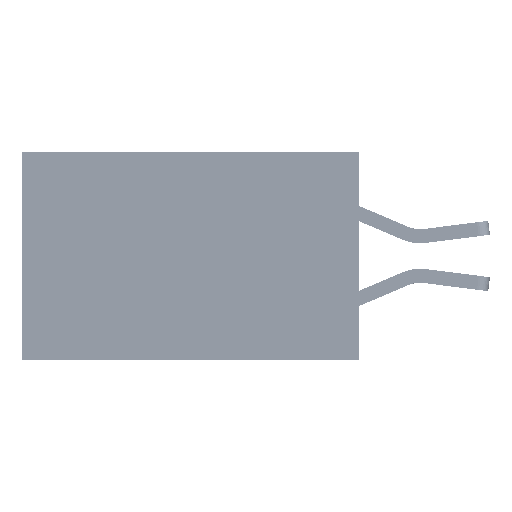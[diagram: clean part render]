
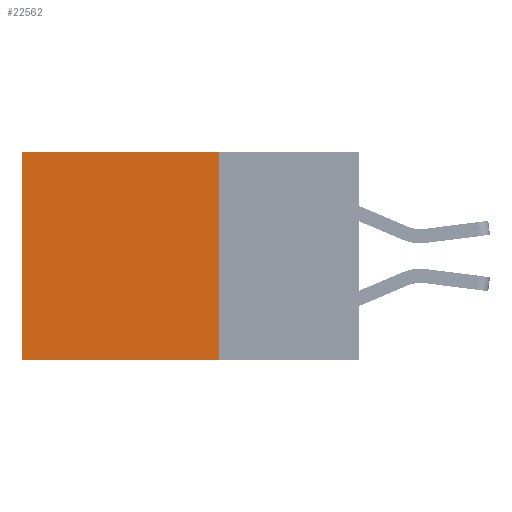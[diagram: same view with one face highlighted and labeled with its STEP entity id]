
A CAD part, left-side view. The second image highlights one B-rep face of the part: STEP entity #22562.
In plain terms, the highlighted planar face has unit normal (-1, 0, 0).
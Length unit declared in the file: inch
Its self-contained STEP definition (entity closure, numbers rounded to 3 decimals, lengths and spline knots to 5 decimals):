
#1526 = AXIS2_PLACEMENT_3D ( 'NONE', #34765, #31621, #42800 ) ;
#2693 = CARTESIAN_POINT ( 'NONE',  ( 0.2875, 0.6, -0.37 ) ) ;
#3317 = LINE ( 'NONE', #44154, #21905 ) ;
#4428 = LINE ( 'NONE', #11513, #46806 ) ;
#4914 = DIRECTION ( 'NONE',  ( 0., 1., 0. ) ) ;
#7636 = VERTEX_POINT ( 'NONE', #46357 ) ;
#10090 = ORIENTED_EDGE ( 'NONE', *, *, #46608, .F. ) ;
#11513 = CARTESIAN_POINT ( 'NONE',  ( 0.2875, 0.25, 0. ) ) ;
#11705 = EDGE_CURVE ( 'NONE', #7636, #19095, #32426, .T. ) ;
#14735 = LINE ( 'NONE', #37545, #40987 ) ;
#15252 = CARTESIAN_POINT ( 'NONE',  ( 0.2875, 0.25, -0.37 ) ) ;
#18324 = ORIENTED_EDGE ( 'NONE', *, *, #11705, .T. ) ;
#18433 = VERTEX_POINT ( 'NONE', #15252 ) ;
#19095 = VERTEX_POINT ( 'NONE', #2693 ) ;
#21905 = VECTOR ( 'NONE', #32981, 39.37008 ) ;
#22562 = ADVANCED_FACE ( 'NONE', ( #23873 ), #35494, .F. ) ;
#23577 = VECTOR ( 'NONE', #43610, 39.37008 ) ;
#23873 = FACE_OUTER_BOUND ( 'NONE', #39299, .T. ) ;
#30512 = DIRECTION ( 'NONE',  ( 0., 0., -1. ) ) ;
#31621 = DIRECTION ( 'NONE',  ( 1., 0., 0. ) ) ;
#32426 = LINE ( 'NONE', #47959, #23577 ) ;
#32981 = DIRECTION ( 'NONE',  ( 0., 1., 0. ) ) ;
#34765 = CARTESIAN_POINT ( 'NONE',  ( 0.2875, 0.25, 0. ) ) ;
#35494 = PLANE ( 'NONE',  #1526 ) ;
#35618 = EDGE_CURVE ( 'NONE', #18433, #19095, #3317, .T. ) ;
#37545 = CARTESIAN_POINT ( 'NONE',  ( 0.2875, 0.25, 0. ) ) ;
#38609 = EDGE_CURVE ( 'NONE', #39523, #7636, #4428, .T. ) ;
#39299 = EDGE_LOOP ( 'NONE', ( #18324, #44200, #10090, #42584 ) ) ;
#39523 = VERTEX_POINT ( 'NONE', #47799 ) ;
#40987 = VECTOR ( 'NONE', #30512, 39.37008 ) ;
#42584 = ORIENTED_EDGE ( 'NONE', *, *, #38609, .T. ) ;
#42800 = DIRECTION ( 'NONE',  ( 0., 0., -1. ) ) ;
#43610 = DIRECTION ( 'NONE',  ( 0., 0., -1. ) ) ;
#44154 = CARTESIAN_POINT ( 'NONE',  ( 0.2875, 0.25, -0.37 ) ) ;
#44200 = ORIENTED_EDGE ( 'NONE', *, *, #35618, .F. ) ;
#46357 = CARTESIAN_POINT ( 'NONE',  ( 0.2875, 0.6, 0. ) ) ;
#46608 = EDGE_CURVE ( 'NONE', #39523, #18433, #14735, .T. ) ;
#46806 = VECTOR ( 'NONE', #4914, 39.37008 ) ;
#47799 = CARTESIAN_POINT ( 'NONE',  ( 0.2875, 0.25, 0. ) ) ;
#47959 = CARTESIAN_POINT ( 'NONE',  ( 0.2875, 0.6, 0. ) ) ;
